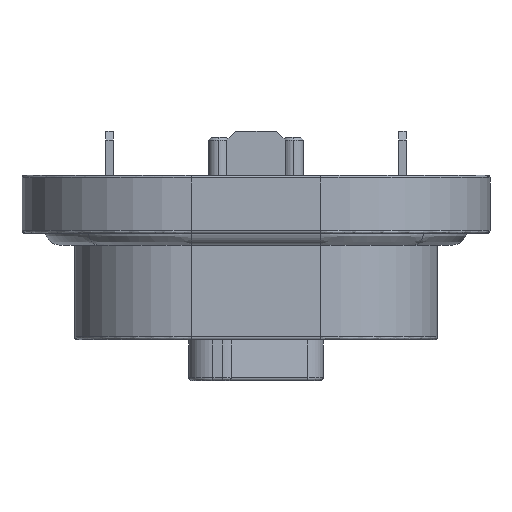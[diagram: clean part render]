
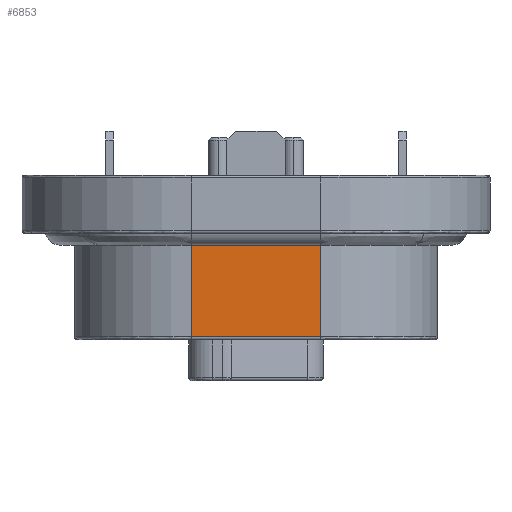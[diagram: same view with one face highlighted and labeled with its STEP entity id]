
A CAD part, left-side view. The second image highlights one B-rep face of the part: STEP entity #6853.
In plain terms, the highlighted planar face has unit normal (-1, 0, 0).
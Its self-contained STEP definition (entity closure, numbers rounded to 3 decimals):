
#203 = EDGE_CURVE ( 'NONE', #21053, #6005, #14849, .T. ) ;
#336 = LINE ( 'NONE', #2286, #19447 ) ;
#568 = FACE_OUTER_BOUND ( 'NONE', #22424, .T. ) ;
#1046 = DIRECTION ( 'NONE',  ( 0., 1., 0. ) ) ;
#2286 = CARTESIAN_POINT ( 'NONE',  ( 36.31, -47.78, 15.059 ) ) ;
#2882 = CARTESIAN_POINT ( 'NONE',  ( 36.31, -50., 15. ) ) ;
#4508 = CARTESIAN_POINT ( 'NONE',  ( 36.31, -52.22, 13.625 ) ) ;
#5221 = CARTESIAN_POINT ( 'NONE',  ( 36.31, -52.22, 10.85 ) ) ;
#5715 = DIRECTION ( 'NONE',  ( 0., 0., 1. ) ) ;
#6005 = VERTEX_POINT ( 'NONE', #8549 ) ;
#6167 = CARTESIAN_POINT ( 'NONE',  ( 36.31, -52.22, 15. ) ) ;
#6853 = ADVANCED_FACE ( 'NONE', ( #568 ), #10990, .F. ) ;
#7223 = CARTESIAN_POINT ( 'NONE',  ( 36.31, -50., 13.625 ) ) ;
#7254 = LINE ( 'NONE', #15920, #15896 ) ;
#8549 = CARTESIAN_POINT ( 'NONE',  ( 36.31, -47.78, 15. ) ) ;
#8693 = ORIENTED_EDGE ( 'NONE', *, *, #14634, .F. ) ;
#9065 = DIRECTION ( 'NONE',  ( 0., 0., -1. ) ) ;
#9313 = DIRECTION ( 'NONE',  ( 0., 0., -1. ) ) ;
#10990 = PLANE ( 'NONE',  #15669 ) ;
#11451 = ORIENTED_EDGE ( 'NONE', *, *, #22484, .F. ) ;
#14199 = VERTEX_POINT ( 'NONE', #16135 ) ;
#14634 = EDGE_CURVE ( 'NONE', #20257, #14199, #7254, .T. ) ;
#14849 = LINE ( 'NONE', #2882, #21463 ) ;
#15669 = AXIS2_PLACEMENT_3D ( 'NONE', #7223, #19315, #9065 ) ;
#15896 = VECTOR ( 'NONE', #18191, 1000. ) ;
#15920 = CARTESIAN_POINT ( 'NONE',  ( 36.31, -50., 10.85 ) ) ;
#16075 = EDGE_CURVE ( 'NONE', #14199, #6005, #336, .T. ) ;
#16135 = CARTESIAN_POINT ( 'NONE',  ( 36.31, -47.78, 10.85 ) ) ;
#16697 = VECTOR ( 'NONE', #9313, 1000. ) ;
#16886 = ORIENTED_EDGE ( 'NONE', *, *, #203, .T. ) ;
#17961 = LINE ( 'NONE', #4508, #16697 ) ;
#18191 = DIRECTION ( 'NONE',  ( 0., 1., 0. ) ) ;
#19315 = DIRECTION ( 'NONE',  ( 1., 0., 0. ) ) ;
#19447 = VECTOR ( 'NONE', #5715, 1000. ) ;
#20257 = VERTEX_POINT ( 'NONE', #5221 ) ;
#21053 = VERTEX_POINT ( 'NONE', #6167 ) ;
#21378 = ORIENTED_EDGE ( 'NONE', *, *, #16075, .F. ) ;
#21463 = VECTOR ( 'NONE', #1046, 1000. ) ;
#22424 = EDGE_LOOP ( 'NONE', ( #16886, #21378, #8693, #11451 ) ) ;
#22484 = EDGE_CURVE ( 'NONE', #21053, #20257, #17961, .T. ) ;
